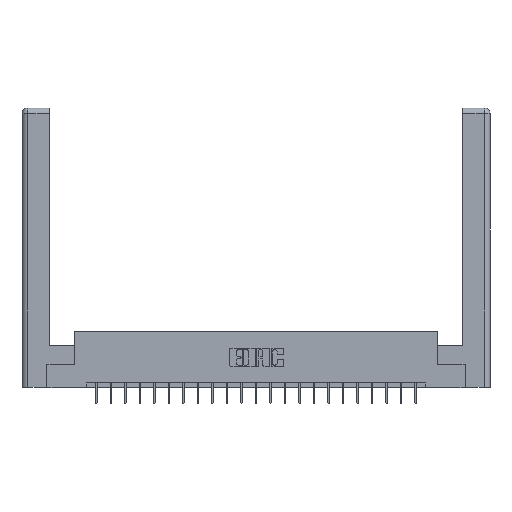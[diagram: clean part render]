
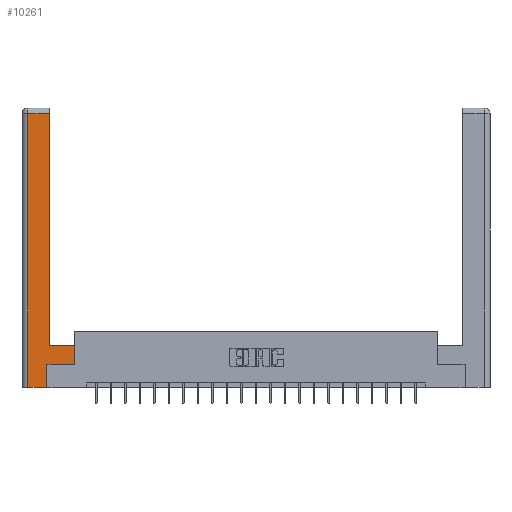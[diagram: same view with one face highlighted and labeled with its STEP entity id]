
A CAD part, top view. The second image highlights one B-rep face of the part: STEP entity #10261.
In plain terms, the highlighted planar face has unit normal (0, 0, 1).
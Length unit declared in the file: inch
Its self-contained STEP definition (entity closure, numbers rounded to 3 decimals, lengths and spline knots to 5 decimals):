
#1959 = LINE ( 'NONE', #17146, #3622 ) ;
#2235 = EDGE_CURVE ( 'NONE', #13388, #8255, #16072, .T. ) ;
#3207 = LINE ( 'NONE', #14301, #8511 ) ;
#3366 = CARTESIAN_POINT ( 'NONE',  ( 0.565, 0.245, 0. ) ) ;
#3399 = LINE ( 'NONE', #13293, #5063 ) ;
#3622 = VECTOR ( 'NONE', #18126, 39.37008 ) ;
#3711 = DIRECTION ( 'NONE',  ( 0., 1., 0. ) ) ;
#3958 = CARTESIAN_POINT ( 'NONE',  ( 0.295, 0.45, 0. ) ) ;
#4408 = AXIS2_PLACEMENT_3D ( 'NONE', #14409, #9029, #21540 ) ;
#4598 = CARTESIAN_POINT ( 'NONE',  ( 0.0615, 0., 0. ) ) ;
#5063 = VECTOR ( 'NONE', #7694, 39.37008 ) ;
#5290 = DIRECTION ( 'NONE',  ( -1., 0., 0. ) ) ;
#7135 = CARTESIAN_POINT ( 'NONE',  ( 0.265, 0.245, 0. ) ) ;
#7207 = ORIENTED_EDGE ( 'NONE', *, *, #21610, .T. ) ;
#7506 = CARTESIAN_POINT ( 'NONE',  ( 0.0615, 2.94, 0. ) ) ;
#7694 = DIRECTION ( 'NONE',  ( 1., 0., 0. ) ) ;
#8253 = EDGE_CURVE ( 'NONE', #8255, #12904, #17606, .T. ) ;
#8255 = VERTEX_POINT ( 'NONE', #13947 ) ;
#8511 = VECTOR ( 'NONE', #12751, 39.37008 ) ;
#8908 = VERTEX_POINT ( 'NONE', #7506 ) ;
#9029 = DIRECTION ( 'NONE',  ( 0., 0., -1. ) ) ;
#9358 = VERTEX_POINT ( 'NONE', #4598 ) ;
#9536 = EDGE_CURVE ( 'NONE', #12904, #20637, #1959, .T. ) ;
#10261 = ADVANCED_FACE ( 'NONE', ( #20929 ), #17926, .F. ) ;
#10751 = VECTOR ( 'NONE', #22109, 39.37008 ) ;
#10883 = VERTEX_POINT ( 'NONE', #11588 ) ;
#11100 = CARTESIAN_POINT ( 'NONE',  ( 0.295, 2.94, 0. ) ) ;
#11588 = CARTESIAN_POINT ( 'NONE',  ( 0.265, 0., 0. ) ) ;
#12169 = CARTESIAN_POINT ( 'NONE',  ( 0.295, 0.45, 0. ) ) ;
#12604 = EDGE_CURVE ( 'NONE', #8908, #9358, #3207, .T. ) ;
#12751 = DIRECTION ( 'NONE',  ( 0., -1., 0. ) ) ;
#12904 = VERTEX_POINT ( 'NONE', #3958 ) ;
#13052 = ORIENTED_EDGE ( 'NONE', *, *, #14036, .T. ) ;
#13153 = VECTOR ( 'NONE', #5290, 39.37008 ) ;
#13286 = CARTESIAN_POINT ( 'NONE',  ( 0.565, 0.45, 0. ) ) ;
#13293 = CARTESIAN_POINT ( 'NONE',  ( 0.565, 0.245, 0. ) ) ;
#13388 = VERTEX_POINT ( 'NONE', #3366 ) ;
#13947 = CARTESIAN_POINT ( 'NONE',  ( 0.565, 0.45, 0. ) ) ;
#14027 = EDGE_LOOP ( 'NONE', ( #16240, #22030, #19775, #7207, #17621, #13052, #15948, #20623 ) ) ;
#14036 = EDGE_CURVE ( 'NONE', #17443, #13388, #3399, .T. ) ;
#14301 = CARTESIAN_POINT ( 'NONE',  ( 0.0615, 0., 0. ) ) ;
#14409 = CARTESIAN_POINT ( 'NONE',  ( 0., 0., 0. ) ) ;
#14465 = CARTESIAN_POINT ( 'NONE',  ( 0.265, 0.245, 0. ) ) ;
#14744 = LINE ( 'NONE', #14465, #17556 ) ;
#14770 = DIRECTION ( 'NONE',  ( -1., 0., 0. ) ) ;
#15948 = ORIENTED_EDGE ( 'NONE', *, *, #2235, .T. ) ;
#16072 = LINE ( 'NONE', #13286, #10751 ) ;
#16240 = ORIENTED_EDGE ( 'NONE', *, *, #9536, .T. ) ;
#17146 = CARTESIAN_POINT ( 'NONE',  ( 0.295, 3., 0. ) ) ;
#17443 = VERTEX_POINT ( 'NONE', #7135 ) ;
#17556 = VECTOR ( 'NONE', #3711, 39.37008 ) ;
#17598 = LINE ( 'NONE', #19016, #18162 ) ;
#17606 = LINE ( 'NONE', #12169, #13153 ) ;
#17621 = ORIENTED_EDGE ( 'NONE', *, *, #22283, .T. ) ;
#17849 = LINE ( 'NONE', #19512, #21501 ) ;
#17926 = PLANE ( 'NONE',  #4408 ) ;
#18126 = DIRECTION ( 'NONE',  ( 0., 1., 0. ) ) ;
#18162 = VECTOR ( 'NONE', #14770, 39.37008 ) ;
#19016 = CARTESIAN_POINT ( 'NONE',  ( 0.0615, 2.94, 0. ) ) ;
#19512 = CARTESIAN_POINT ( 'NONE',  ( 0.265, 0., 0. ) ) ;
#19750 = EDGE_CURVE ( 'NONE', #20637, #8908, #17598, .T. ) ;
#19775 = ORIENTED_EDGE ( 'NONE', *, *, #12604, .T. ) ;
#20623 = ORIENTED_EDGE ( 'NONE', *, *, #8253, .T. ) ;
#20637 = VERTEX_POINT ( 'NONE', #11100 ) ;
#20929 = FACE_OUTER_BOUND ( 'NONE', #14027, .T. ) ;
#21469 = DIRECTION ( 'NONE',  ( 1., 0., 0. ) ) ;
#21501 = VECTOR ( 'NONE', #21469, 39.37008 ) ;
#21540 = DIRECTION ( 'NONE',  ( -1., 0., 0. ) ) ;
#21610 = EDGE_CURVE ( 'NONE', #9358, #10883, #17849, .T. ) ;
#22030 = ORIENTED_EDGE ( 'NONE', *, *, #19750, .T. ) ;
#22109 = DIRECTION ( 'NONE',  ( 0., 1., 0. ) ) ;
#22283 = EDGE_CURVE ( 'NONE', #10883, #17443, #14744, .T. ) ;
